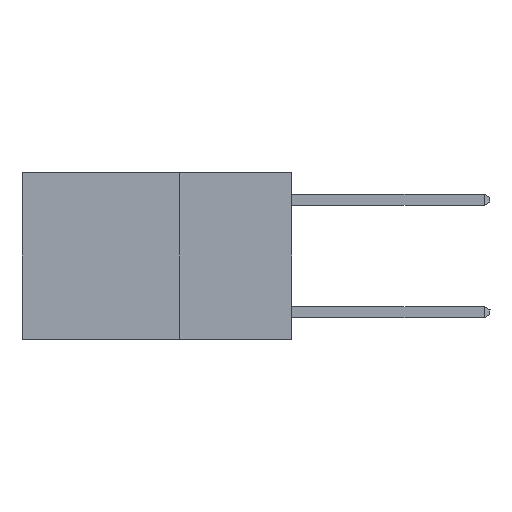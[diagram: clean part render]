
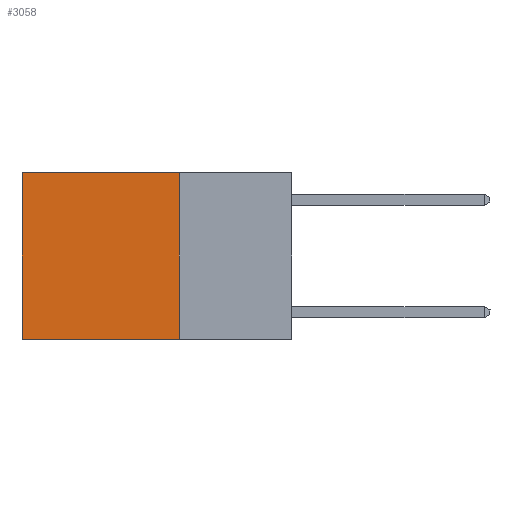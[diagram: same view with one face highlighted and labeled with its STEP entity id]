
A CAD part, left-side view. The second image highlights one B-rep face of the part: STEP entity #3058.
In plain terms, the highlighted planar face has unit normal (-1, 0, 0).
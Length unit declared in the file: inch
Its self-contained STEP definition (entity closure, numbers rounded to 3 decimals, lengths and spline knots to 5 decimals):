
#1015 = EDGE_CURVE ( 'NONE', #14781, #14399, #16979, .T. ) ;
#1889 = PLANE ( 'NONE',  #2237 ) ;
#2237 = AXIS2_PLACEMENT_3D ( 'NONE', #13032, #14528, #5178 ) ;
#3058 = ADVANCED_FACE ( 'NONE', ( #5721 ), #1889, .F. ) ;
#3411 = ORIENTED_EDGE ( 'NONE', *, *, #4363, .F. ) ;
#3569 = ORIENTED_EDGE ( 'NONE', *, *, #16499, .F. ) ;
#4363 = EDGE_CURVE ( 'NONE', #18917, #10711, #19138, .T. ) ;
#5014 = CARTESIAN_POINT ( 'NONE',  ( 0.2625, 0.25, 0. ) ) ;
#5178 = DIRECTION ( 'NONE',  ( 0., 0., -1. ) ) ;
#5721 = FACE_OUTER_BOUND ( 'NONE', #20152, .T. ) ;
#5921 = CARTESIAN_POINT ( 'NONE',  ( 0.2625, 0.6, -0.37 ) ) ;
#6471 = CARTESIAN_POINT ( 'NONE',  ( 0.2625, 0.6, 0. ) ) ;
#6959 = DIRECTION ( 'NONE',  ( 0., 0., -1. ) ) ;
#7220 = VECTOR ( 'NONE', #17433, 39.37008 ) ;
#7267 = EDGE_CURVE ( 'NONE', #14399, #10711, #18496, .T. ) ;
#8419 = DIRECTION ( 'NONE',  ( 0., 1., 0. ) ) ;
#8529 = CARTESIAN_POINT ( 'NONE',  ( 0.2625, 0.25, 0. ) ) ;
#9693 = CARTESIAN_POINT ( 'NONE',  ( 0.2625, 0.25, -0.37 ) ) ;
#10711 = VERTEX_POINT ( 'NONE', #5921 ) ;
#13032 = CARTESIAN_POINT ( 'NONE',  ( 0.2625, 0.25, 0. ) ) ;
#14399 = VERTEX_POINT ( 'NONE', #6471 ) ;
#14528 = DIRECTION ( 'NONE',  ( 1., 0., 0. ) ) ;
#14781 = VERTEX_POINT ( 'NONE', #15170 ) ;
#15170 = CARTESIAN_POINT ( 'NONE',  ( 0.2625, 0.25, 0. ) ) ;
#16003 = LINE ( 'NONE', #5014, #7220 ) ;
#16285 = CARTESIAN_POINT ( 'NONE',  ( 0.2625, 0.6, 0. ) ) ;
#16499 = EDGE_CURVE ( 'NONE', #14781, #18917, #16003, .T. ) ;
#16777 = VECTOR ( 'NONE', #8419, 39.37008 ) ;
#16979 = LINE ( 'NONE', #8529, #16777 ) ;
#17433 = DIRECTION ( 'NONE',  ( 0., 0., -1. ) ) ;
#18254 = CARTESIAN_POINT ( 'NONE',  ( 0.2625, 0.25, -0.37 ) ) ;
#18326 = ORIENTED_EDGE ( 'NONE', *, *, #1015, .T. ) ;
#18459 = VECTOR ( 'NONE', #6959, 39.37008 ) ;
#18496 = LINE ( 'NONE', #16285, #18459 ) ;
#18917 = VERTEX_POINT ( 'NONE', #18254 ) ;
#19138 = LINE ( 'NONE', #9693, #19630 ) ;
#19462 = ORIENTED_EDGE ( 'NONE', *, *, #7267, .T. ) ;
#19630 = VECTOR ( 'NONE', #20189, 39.37008 ) ;
#20152 = EDGE_LOOP ( 'NONE', ( #19462, #3411, #3569, #18326 ) ) ;
#20189 = DIRECTION ( 'NONE',  ( 0., 1., 0. ) ) ;
